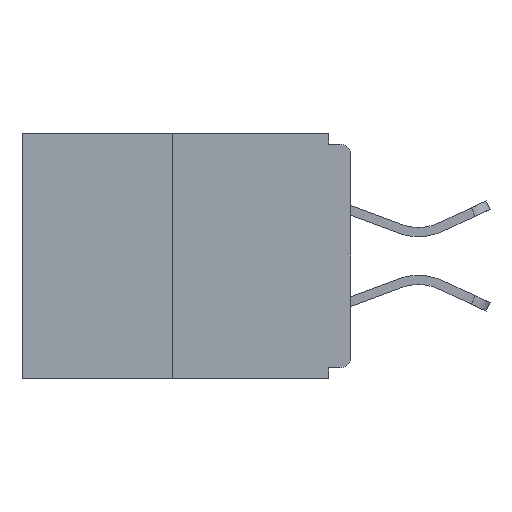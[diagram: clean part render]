
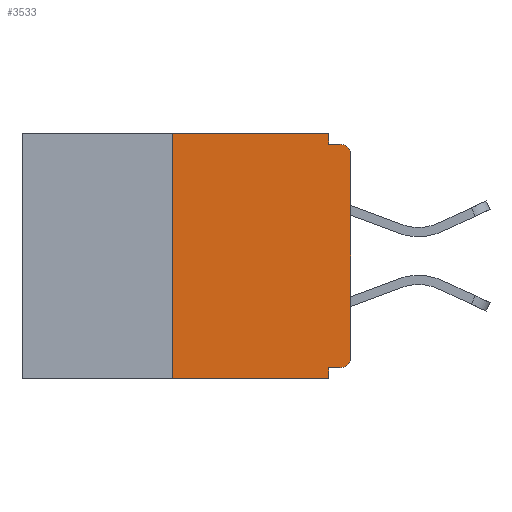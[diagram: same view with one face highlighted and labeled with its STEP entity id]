
A CAD part, left-side view. The second image highlights one B-rep face of the part: STEP entity #3533.
In plain terms, the highlighted planar face has unit normal (-1, 0, 0).
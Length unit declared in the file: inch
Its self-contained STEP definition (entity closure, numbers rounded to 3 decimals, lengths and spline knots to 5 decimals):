
#156 = CARTESIAN_POINT ( 'NONE',  ( 0., 0.015, -0.313 ) ) ;
#191 = CARTESIAN_POINT ( 'NONE',  ( 0., 0.46, -0.343 ) ) ;
#352 = CARTESIAN_POINT ( 'NONE',  ( 0., 0.46, 0. ) ) ;
#376 = VECTOR ( 'NONE', #2785, 39.37008 ) ;
#482 = EDGE_CURVE ( 'NONE', #11875, #2735, #14512, .T. ) ;
#569 = CARTESIAN_POINT ( 'NONE',  ( 0., 0.46, 0. ) ) ;
#591 = CARTESIAN_POINT ( 'NONE',  ( 0., 0., 0. ) ) ;
#1101 = AXIS2_PLACEMENT_3D ( 'NONE', #4323, #7775, #9007 ) ;
#1266 = ORIENTED_EDGE ( 'NONE', *, *, #9591, .T. ) ;
#1661 = CARTESIAN_POINT ( 'NONE',  ( 0., 0., -0.03 ) ) ;
#2036 = AXIS2_PLACEMENT_3D ( 'NONE', #569, #11279, #3086 ) ;
#2281 = VERTEX_POINT ( 'NONE', #6205 ) ;
#2398 = EDGE_CURVE ( 'NONE', #2281, #11875, #4459, .T. ) ;
#2709 = CARTESIAN_POINT ( 'NONE',  ( 0., 0., -0.313 ) ) ;
#2722 = DIRECTION ( 'NONE',  ( 0., -1., 0. ) ) ;
#2735 = VERTEX_POINT ( 'NONE', #14962 ) ;
#2785 = DIRECTION ( 'NONE',  ( 0., 0., -1. ) ) ;
#3086 = DIRECTION ( 'NONE',  ( 0., 0., -1. ) ) ;
#3271 = EDGE_CURVE ( 'NONE', #14365, #12441, #4755, .T. ) ;
#3376 = EDGE_LOOP ( 'NONE', ( #11989, #12253, #8248, #8748, #10962, #6954, #12925, #1266, #3608, #7781 ) ) ;
#3396 = VECTOR ( 'NONE', #10038, 39.37008 ) ;
#3463 = EDGE_CURVE ( 'NONE', #4558, #2281, #11002, .T. ) ;
#3518 = AXIS2_PLACEMENT_3D ( 'NONE', #156, #13108, #6102 ) ;
#3533 = ADVANCED_FACE ( 'NONE', ( #9164 ), #7795, .F. ) ;
#3608 = ORIENTED_EDGE ( 'NONE', *, *, #5911, .F. ) ;
#3729 = VECTOR ( 'NONE', #6932, 39.37008 ) ;
#3767 = DIRECTION ( 'NONE',  ( 0., -1., 0. ) ) ;
#3780 = LINE ( 'NONE', #591, #3396 ) ;
#3834 = VERTEX_POINT ( 'NONE', #6621 ) ;
#4323 = CARTESIAN_POINT ( 'NONE',  ( 0., 0.015, -0.03 ) ) ;
#4459 = LINE ( 'NONE', #352, #14501 ) ;
#4555 = VECTOR ( 'NONE', #7143, 39.37008 ) ;
#4558 = VERTEX_POINT ( 'NONE', #14061 ) ;
#4755 = CIRCLE ( 'NONE', #3518, 0.015 ) ;
#5512 = CARTESIAN_POINT ( 'NONE',  ( 0., 0.031, -0.328 ) ) ;
#5911 = EDGE_CURVE ( 'NONE', #2735, #14835, #14233, .T. ) ;
#6102 = DIRECTION ( 'NONE',  ( 0., 0., -1. ) ) ;
#6205 = CARTESIAN_POINT ( 'NONE',  ( 0., 0.25, 0. ) ) ;
#6305 = CARTESIAN_POINT ( 'NONE',  ( 0., 0.031, -0.343 ) ) ;
#6621 = CARTESIAN_POINT ( 'NONE',  ( 0., 0.031, -0.343 ) ) ;
#6932 = DIRECTION ( 'NONE',  ( 0., 0., -1. ) ) ;
#6954 = ORIENTED_EDGE ( 'NONE', *, *, #3271, .T. ) ;
#7143 = DIRECTION ( 'NONE',  ( 0., -1., 0. ) ) ;
#7320 = EDGE_CURVE ( 'NONE', #12441, #11856, #3780, .T. ) ;
#7671 = CARTESIAN_POINT ( 'NONE',  ( 0., 0.015, -0.328 ) ) ;
#7775 = DIRECTION ( 'NONE',  ( -1., 0., 0. ) ) ;
#7781 = ORIENTED_EDGE ( 'NONE', *, *, #482, .F. ) ;
#7795 = PLANE ( 'NONE',  #2036 ) ;
#8248 = ORIENTED_EDGE ( 'NONE', *, *, #13188, .T. ) ;
#8748 = ORIENTED_EDGE ( 'NONE', *, *, #13085, .F. ) ;
#8877 = DIRECTION ( 'NONE',  ( 0., 0., 1. ) ) ;
#9007 = DIRECTION ( 'NONE',  ( 0., 0., -1. ) ) ;
#9039 = CARTESIAN_POINT ( 'NONE',  ( 0., 0.031, 0. ) ) ;
#9164 = FACE_OUTER_BOUND ( 'NONE', #3376, .T. ) ;
#9591 = EDGE_CURVE ( 'NONE', #11856, #14835, #9626, .T. ) ;
#9598 = VERTEX_POINT ( 'NONE', #5512 ) ;
#9626 = CIRCLE ( 'NONE', #1101, 0.015 ) ;
#9910 = CARTESIAN_POINT ( 'NONE',  ( 0., 0.031, 0. ) ) ;
#10038 = DIRECTION ( 'NONE',  ( 0., 0., 1. ) ) ;
#10962 = ORIENTED_EDGE ( 'NONE', *, *, #11370, .F. ) ;
#11002 = LINE ( 'NONE', #14678, #13707 ) ;
#11279 = DIRECTION ( 'NONE',  ( 1., 0., 0. ) ) ;
#11370 = EDGE_CURVE ( 'NONE', #14365, #9598, #14368, .T. ) ;
#11739 = CARTESIAN_POINT ( 'NONE',  ( 0., 0., -0.015 ) ) ;
#11856 = VERTEX_POINT ( 'NONE', #1661 ) ;
#11875 = VERTEX_POINT ( 'NONE', #9910 ) ;
#11962 = LINE ( 'NONE', #191, #13217 ) ;
#11989 = ORIENTED_EDGE ( 'NONE', *, *, #2398, .F. ) ;
#12253 = ORIENTED_EDGE ( 'NONE', *, *, #3463, .F. ) ;
#12441 = VERTEX_POINT ( 'NONE', #2709 ) ;
#12925 = ORIENTED_EDGE ( 'NONE', *, *, #7320, .T. ) ;
#12958 = CARTESIAN_POINT ( 'NONE',  ( 0., 0., -0.328 ) ) ;
#13085 = EDGE_CURVE ( 'NONE', #9598, #3834, #13594, .T. ) ;
#13108 = DIRECTION ( 'NONE',  ( -1., 0., 0. ) ) ;
#13188 = EDGE_CURVE ( 'NONE', #4558, #3834, #11962, .T. ) ;
#13217 = VECTOR ( 'NONE', #3767, 39.37008 ) ;
#13594 = LINE ( 'NONE', #6305, #376 ) ;
#13707 = VECTOR ( 'NONE', #8877, 39.37008 ) ;
#14061 = CARTESIAN_POINT ( 'NONE',  ( 0., 0.25, -0.343 ) ) ;
#14233 = LINE ( 'NONE', #11739, #4555 ) ;
#14365 = VERTEX_POINT ( 'NONE', #7671 ) ;
#14368 = LINE ( 'NONE', #12958, #14713 ) ;
#14501 = VECTOR ( 'NONE', #2722, 39.37008 ) ;
#14512 = LINE ( 'NONE', #9039, #3729 ) ;
#14678 = CARTESIAN_POINT ( 'NONE',  ( 0., 0.25, 0. ) ) ;
#14679 = CARTESIAN_POINT ( 'NONE',  ( 0., 0.015, -0.015 ) ) ;
#14713 = VECTOR ( 'NONE', #14961, 39.37008 ) ;
#14835 = VERTEX_POINT ( 'NONE', #14679 ) ;
#14961 = DIRECTION ( 'NONE',  ( 0., 1., 0. ) ) ;
#14962 = CARTESIAN_POINT ( 'NONE',  ( 0., 0.031, -0.015 ) ) ;
